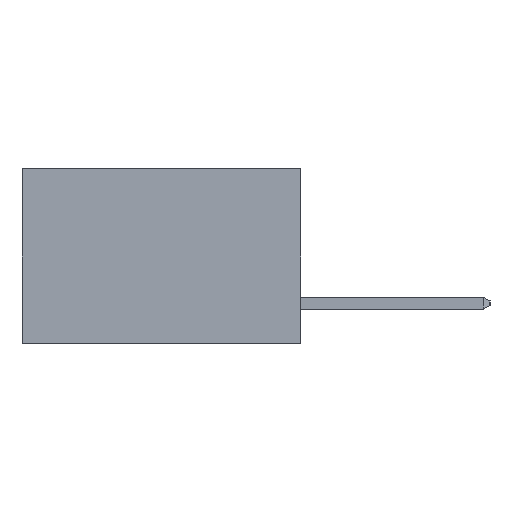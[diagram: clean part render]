
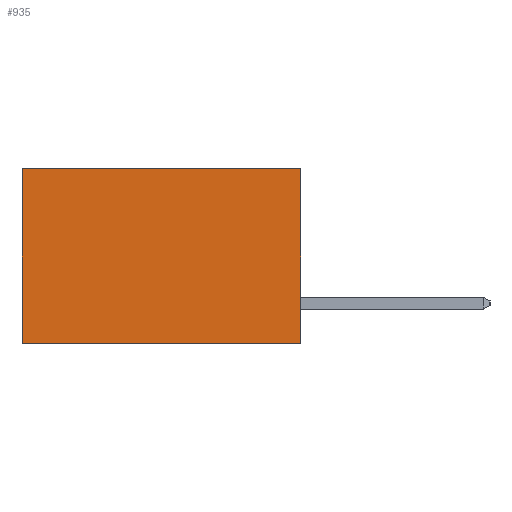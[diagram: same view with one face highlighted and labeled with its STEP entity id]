
A CAD part, left-side view. The second image highlights one B-rep face of the part: STEP entity #935.
In plain terms, the highlighted planar face has unit normal (-1, 0, 0).
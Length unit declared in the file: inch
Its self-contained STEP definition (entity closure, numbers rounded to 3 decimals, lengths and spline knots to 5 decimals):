
#78 = FACE_OUTER_BOUND ( 'NONE', #11313, .T. ) ;
#935 = ADVANCED_FACE ( 'NONE', ( #78 ), #16874, .F. ) ;
#1464 = ORIENTED_EDGE ( 'NONE', *, *, #15054, .T. ) ;
#1737 = CARTESIAN_POINT ( 'NONE',  ( 0.277, 0.59, 0. ) ) ;
#3150 = VERTEX_POINT ( 'NONE', #3293 ) ;
#3293 = CARTESIAN_POINT ( 'NONE',  ( 0.277, 0., -0.37 ) ) ;
#3991 = DIRECTION ( 'NONE',  ( 0., 0., -1. ) ) ;
#4035 = VECTOR ( 'NONE', #7647, 39.37008 ) ;
#5361 = EDGE_CURVE ( 'NONE', #6215, #3150, #15764, .T. ) ;
#5921 = VERTEX_POINT ( 'NONE', #1737 ) ;
#6215 = VERTEX_POINT ( 'NONE', #11087 ) ;
#6328 = VECTOR ( 'NONE', #3991, 39.37008 ) ;
#7647 = DIRECTION ( 'NONE',  ( 0., 1., 0. ) ) ;
#7893 = ORIENTED_EDGE ( 'NONE', *, *, #11286, .T. ) ;
#7945 = CARTESIAN_POINT ( 'NONE',  ( 0.277, 0., 0. ) ) ;
#8242 = VECTOR ( 'NONE', #15088, 39.37008 ) ;
#9084 = CARTESIAN_POINT ( 'NONE',  ( 0.277, 0., -0.37 ) ) ;
#10506 = ORIENTED_EDGE ( 'NONE', *, *, #5361, .F. ) ;
#10700 = AXIS2_PLACEMENT_3D ( 'NONE', #14959, #12546, #16586 ) ;
#10973 = EDGE_CURVE ( 'NONE', #3150, #14579, #11673, .T. ) ;
#11087 = CARTESIAN_POINT ( 'NONE',  ( 0.277, 0., 0. ) ) ;
#11286 = EDGE_CURVE ( 'NONE', #5921, #14579, #14294, .T. ) ;
#11313 = EDGE_LOOP ( 'NONE', ( #7893, #17329, #10506, #1464 ) ) ;
#11673 = LINE ( 'NONE', #9084, #4035 ) ;
#12546 = DIRECTION ( 'NONE',  ( 1., 0., 0. ) ) ;
#12576 = CARTESIAN_POINT ( 'NONE',  ( 0.277, 0.59, -0.37 ) ) ;
#14294 = LINE ( 'NONE', #12576, #6328 ) ;
#14579 = VERTEX_POINT ( 'NONE', #16822 ) ;
#14959 = CARTESIAN_POINT ( 'NONE',  ( 0.277, 0., -0.37 ) ) ;
#15054 = EDGE_CURVE ( 'NONE', #6215, #5921, #17669, .T. ) ;
#15060 = DIRECTION ( 'NONE',  ( 0., 1., 0. ) ) ;
#15088 = DIRECTION ( 'NONE',  ( 0., 0., -1. ) ) ;
#15590 = CARTESIAN_POINT ( 'NONE',  ( 0.277, 0., -0.37 ) ) ;
#15764 = LINE ( 'NONE', #15590, #8242 ) ;
#16586 = DIRECTION ( 'NONE',  ( 0., 0., -1. ) ) ;
#16822 = CARTESIAN_POINT ( 'NONE',  ( 0.277, 0.59, -0.37 ) ) ;
#16874 = PLANE ( 'NONE',  #10700 ) ;
#17229 = VECTOR ( 'NONE', #15060, 39.37008 ) ;
#17329 = ORIENTED_EDGE ( 'NONE', *, *, #10973, .F. ) ;
#17669 = LINE ( 'NONE', #7945, #17229 ) ;
